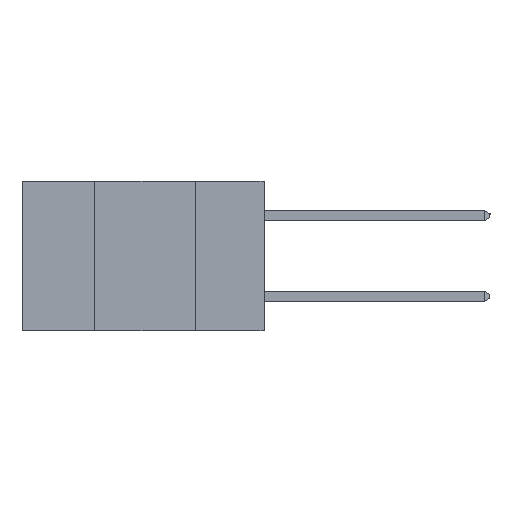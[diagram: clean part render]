
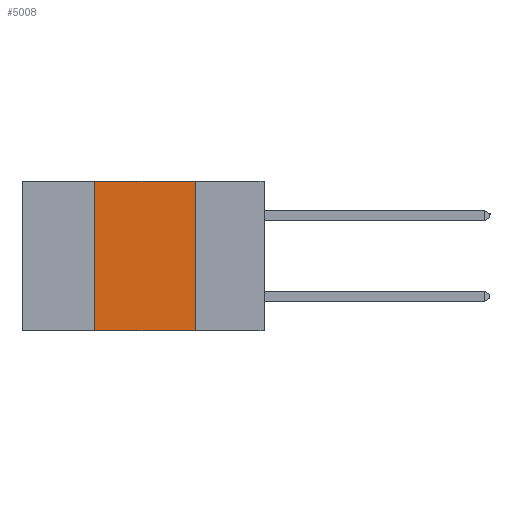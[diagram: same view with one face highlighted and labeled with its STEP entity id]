
A CAD part, left-side view. The second image highlights one B-rep face of the part: STEP entity #5008.
In plain terms, the highlighted planar face has unit normal (-1, 0, 0).
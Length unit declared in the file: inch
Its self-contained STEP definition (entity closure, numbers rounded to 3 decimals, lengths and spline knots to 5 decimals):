
#329 = VECTOR ( 'NONE', #10978, 39.37008 ) ;
#506 = EDGE_CURVE ( 'NONE', #15541, #9434, #615, .T. ) ;
#615 = LINE ( 'NONE', #15431, #13655 ) ;
#997 = VECTOR ( 'NONE', #14862, 39.37008 ) ;
#1165 = DIRECTION ( 'NONE',  ( 0., 0., -1. ) ) ;
#1167 = CARTESIAN_POINT ( 'NONE',  ( 0., 0.6, -0.37 ) ) ;
#1348 = EDGE_LOOP ( 'NONE', ( #11218, #8153, #5659, #3400 ) ) ;
#2341 = VERTEX_POINT ( 'NONE', #11766 ) ;
#3400 = ORIENTED_EDGE ( 'NONE', *, *, #11719, .T. ) ;
#4325 = AXIS2_PLACEMENT_3D ( 'NONE', #7421, #12270, #1165 ) ;
#4759 = DIRECTION ( 'NONE',  ( 0., -1., 0. ) ) ;
#5008 = ADVANCED_FACE ( 'NONE', ( #12435 ), #7496, .F. ) ;
#5019 = CARTESIAN_POINT ( 'NONE',  ( 0., 0.17, -0.37 ) ) ;
#5286 = EDGE_CURVE ( 'NONE', #2341, #11949, #7745, .T. ) ;
#5659 = ORIENTED_EDGE ( 'NONE', *, *, #506, .F. ) ;
#6543 = CARTESIAN_POINT ( 'NONE',  ( 0., 0.17, -0.37 ) ) ;
#7095 = LINE ( 'NONE', #12026, #11822 ) ;
#7421 = CARTESIAN_POINT ( 'NONE',  ( 0., 0.6, 0. ) ) ;
#7496 = PLANE ( 'NONE',  #4325 ) ;
#7745 = LINE ( 'NONE', #5019, #997 ) ;
#7804 = EDGE_CURVE ( 'NONE', #9434, #2341, #7095, .T. ) ;
#8153 = ORIENTED_EDGE ( 'NONE', *, *, #7804, .F. ) ;
#8631 = LINE ( 'NONE', #1167, #329 ) ;
#9434 = VERTEX_POINT ( 'NONE', #14642 ) ;
#10978 = DIRECTION ( 'NONE',  ( 0., -1., 0. ) ) ;
#11218 = ORIENTED_EDGE ( 'NONE', *, *, #5286, .F. ) ;
#11719 = EDGE_CURVE ( 'NONE', #15541, #11949, #8631, .T. ) ;
#11766 = CARTESIAN_POINT ( 'NONE',  ( 0., 0.17, 0. ) ) ;
#11822 = VECTOR ( 'NONE', #4759, 39.37008 ) ;
#11949 = VERTEX_POINT ( 'NONE', #6543 ) ;
#12026 = CARTESIAN_POINT ( 'NONE',  ( 0., 0.6, 0. ) ) ;
#12270 = DIRECTION ( 'NONE',  ( 1., 0., 0. ) ) ;
#12435 = FACE_OUTER_BOUND ( 'NONE', #1348, .T. ) ;
#13655 = VECTOR ( 'NONE', #15270, 39.37008 ) ;
#14476 = CARTESIAN_POINT ( 'NONE',  ( 0., 0.42, -0.37 ) ) ;
#14642 = CARTESIAN_POINT ( 'NONE',  ( 0., 0.42, 0. ) ) ;
#14862 = DIRECTION ( 'NONE',  ( 0., 0., -1. ) ) ;
#15270 = DIRECTION ( 'NONE',  ( 0., 0., 1. ) ) ;
#15431 = CARTESIAN_POINT ( 'NONE',  ( 0., 0.42, -0.37 ) ) ;
#15541 = VERTEX_POINT ( 'NONE', #14476 ) ;
